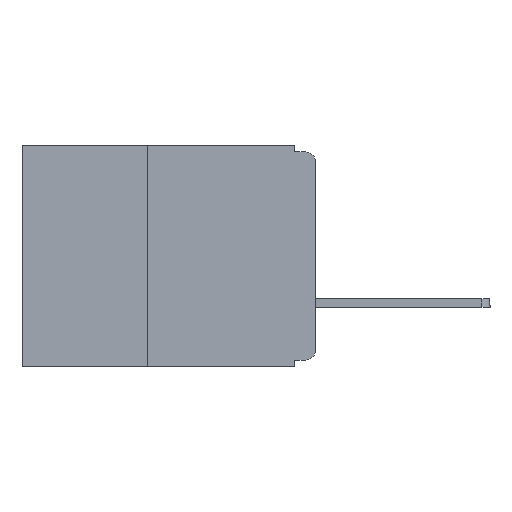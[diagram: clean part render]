
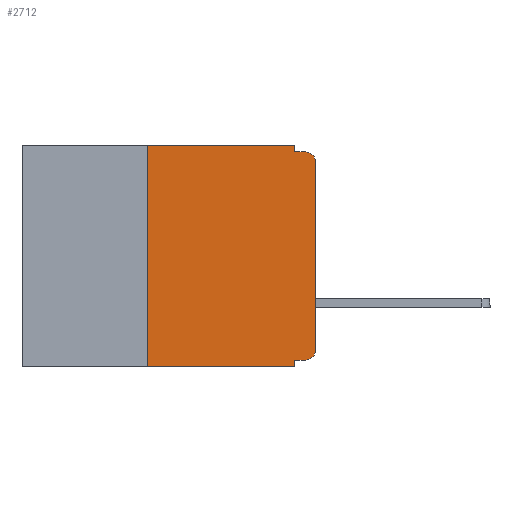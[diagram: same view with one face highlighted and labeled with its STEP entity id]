
A CAD part, left-side view. The second image highlights one B-rep face of the part: STEP entity #2712.
In plain terms, the highlighted planar face has unit normal (-1, 0, 0).
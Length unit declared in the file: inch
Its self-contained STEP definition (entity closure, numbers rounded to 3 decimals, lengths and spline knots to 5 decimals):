
#52 = VECTOR ( 'NONE', #12586, 39.37008 ) ;
#129 = ORIENTED_EDGE ( 'NONE', *, *, #21061, .T. ) ;
#173 = CARTESIAN_POINT ( 'NONE',  ( 0., 0.437, -0.33 ) ) ;
#361 = CARTESIAN_POINT ( 'NONE',  ( 0., 0., -0.305 ) ) ;
#494 = EDGE_CURVE ( 'NONE', #7946, #4971, #5809, .T. ) ;
#537 = EDGE_CURVE ( 'NONE', #8335, #21397, #9353, .T. ) ;
#697 = LINE ( 'NONE', #15711, #18582 ) ;
#946 = EDGE_LOOP ( 'NONE', ( #16681, #20934, #6459, #18796, #12534, #5218, #9068, #18330, #2306, #129 ) ) ;
#1603 = LINE ( 'NONE', #14274, #14905 ) ;
#1838 = DIRECTION ( 'NONE',  ( 0., 0., -1. ) ) ;
#2045 = VERTEX_POINT ( 'NONE', #22030 ) ;
#2090 = CARTESIAN_POINT ( 'NONE',  ( 0., 0.25, 0. ) ) ;
#2243 = CARTESIAN_POINT ( 'NONE',  ( 0., 0.031, -0.32 ) ) ;
#2306 = ORIENTED_EDGE ( 'NONE', *, *, #6783, .F. ) ;
#2453 = EDGE_CURVE ( 'NONE', #14867, #21746, #14072, .T. ) ;
#2712 = ADVANCED_FACE ( 'NONE', ( #4031 ), #21261, .F. ) ;
#3040 = VERTEX_POINT ( 'NONE', #17098 ) ;
#3292 = VECTOR ( 'NONE', #3670, 39.37008 ) ;
#3362 = AXIS2_PLACEMENT_3D ( 'NONE', #14103, #13727, #13540 ) ;
#3487 = LINE ( 'NONE', #14834, #12226 ) ;
#3670 = DIRECTION ( 'NONE',  ( 0., -1., 0. ) ) ;
#4031 = FACE_OUTER_BOUND ( 'NONE', #946, .T. ) ;
#4135 = CARTESIAN_POINT ( 'NONE',  ( 0., 0.015, -0.01 ) ) ;
#4971 = VERTEX_POINT ( 'NONE', #4135 ) ;
#5218 = ORIENTED_EDGE ( 'NONE', *, *, #537, .F. ) ;
#5604 = CARTESIAN_POINT ( 'NONE',  ( 0., 0., -0.32 ) ) ;
#5809 = CIRCLE ( 'NONE', #3362, 0.015 ) ;
#6049 = VECTOR ( 'NONE', #6880, 39.37008 ) ;
#6459 = ORIENTED_EDGE ( 'NONE', *, *, #9477, .F. ) ;
#6531 = CARTESIAN_POINT ( 'NONE',  ( 0., 0.031, -0.01 ) ) ;
#6783 = EDGE_CURVE ( 'NONE', #2045, #14867, #19770, .T. ) ;
#6880 = DIRECTION ( 'NONE',  ( 0., 0., 1. ) ) ;
#7089 = CARTESIAN_POINT ( 'NONE',  ( 0., 0.031, -0.33 ) ) ;
#7946 = VERTEX_POINT ( 'NONE', #16350 ) ;
#7999 = LINE ( 'NONE', #173, #3292 ) ;
#8028 = EDGE_CURVE ( 'NONE', #3040, #13187, #3487, .T. ) ;
#8335 = VERTEX_POINT ( 'NONE', #10473 ) ;
#9068 = ORIENTED_EDGE ( 'NONE', *, *, #12795, .T. ) ;
#9353 = LINE ( 'NONE', #11539, #52 ) ;
#9477 = EDGE_CURVE ( 'NONE', #13187, #4971, #697, .T. ) ;
#9934 = CARTESIAN_POINT ( 'NONE',  ( 0., 0.015, -0.305 ) ) ;
#10473 = CARTESIAN_POINT ( 'NONE',  ( 0., 0.25, -0.33 ) ) ;
#10648 = LINE ( 'NONE', #12018, #6049 ) ;
#11206 = CARTESIAN_POINT ( 'NONE',  ( 0., 0.031, -0.33 ) ) ;
#11539 = CARTESIAN_POINT ( 'NONE',  ( 0., 0.25, -0.33 ) ) ;
#11648 = DIRECTION ( 'NONE',  ( 0., 0., -1. ) ) ;
#11749 = VERTEX_POINT ( 'NONE', #361 ) ;
#12018 = CARTESIAN_POINT ( 'NONE',  ( 0., 0., 0. ) ) ;
#12226 = VECTOR ( 'NONE', #16586, 39.37008 ) ;
#12534 = ORIENTED_EDGE ( 'NONE', *, *, #14180, .F. ) ;
#12586 = DIRECTION ( 'NONE',  ( 0., 0., 1. ) ) ;
#12795 = EDGE_CURVE ( 'NONE', #8335, #21746, #7999, .T. ) ;
#13187 = VERTEX_POINT ( 'NONE', #6531 ) ;
#13533 = VECTOR ( 'NONE', #1838, 39.37008 ) ;
#13540 = DIRECTION ( 'NONE',  ( 0., 0., -1. ) ) ;
#13727 = DIRECTION ( 'NONE',  ( -1., 0., 0. ) ) ;
#14072 = LINE ( 'NONE', #7089, #13533 ) ;
#14103 = CARTESIAN_POINT ( 'NONE',  ( 0., 0.015, -0.025 ) ) ;
#14180 = EDGE_CURVE ( 'NONE', #21397, #3040, #1603, .T. ) ;
#14274 = CARTESIAN_POINT ( 'NONE',  ( 0., 0.437, 0. ) ) ;
#14684 = VECTOR ( 'NONE', #19457, 39.37008 ) ;
#14834 = CARTESIAN_POINT ( 'NONE',  ( 0., 0.031, 0. ) ) ;
#14867 = VERTEX_POINT ( 'NONE', #2243 ) ;
#14905 = VECTOR ( 'NONE', #16042, 39.37008 ) ;
#14994 = CIRCLE ( 'NONE', #15205, 0.015 ) ;
#15205 = AXIS2_PLACEMENT_3D ( 'NONE', #9934, #21839, #11648 ) ;
#15711 = CARTESIAN_POINT ( 'NONE',  ( 0., 0., -0.01 ) ) ;
#16042 = DIRECTION ( 'NONE',  ( 0., -1., 0. ) ) ;
#16350 = CARTESIAN_POINT ( 'NONE',  ( 0., 0., -0.025 ) ) ;
#16586 = DIRECTION ( 'NONE',  ( 0., 0., -1. ) ) ;
#16681 = ORIENTED_EDGE ( 'NONE', *, *, #22037, .T. ) ;
#17098 = CARTESIAN_POINT ( 'NONE',  ( 0., 0.031, 0. ) ) ;
#18330 = ORIENTED_EDGE ( 'NONE', *, *, #2453, .F. ) ;
#18582 = VECTOR ( 'NONE', #19106, 39.37008 ) ;
#18796 = ORIENTED_EDGE ( 'NONE', *, *, #8028, .F. ) ;
#19106 = DIRECTION ( 'NONE',  ( 0., -1., 0. ) ) ;
#19457 = DIRECTION ( 'NONE',  ( 0., 1., 0. ) ) ;
#19770 = LINE ( 'NONE', #5604, #14684 ) ;
#20934 = ORIENTED_EDGE ( 'NONE', *, *, #494, .T. ) ;
#21061 = EDGE_CURVE ( 'NONE', #2045, #11749, #14994, .T. ) ;
#21108 = DIRECTION ( 'NONE',  ( 1., 0., 0. ) ) ;
#21186 = CARTESIAN_POINT ( 'NONE',  ( 0., 0.437, 0. ) ) ;
#21261 = PLANE ( 'NONE',  #22276 ) ;
#21397 = VERTEX_POINT ( 'NONE', #2090 ) ;
#21746 = VERTEX_POINT ( 'NONE', #11206 ) ;
#21839 = DIRECTION ( 'NONE',  ( -1., 0., 0. ) ) ;
#21990 = DIRECTION ( 'NONE',  ( 0., 0., -1. ) ) ;
#22030 = CARTESIAN_POINT ( 'NONE',  ( 0., 0.015, -0.32 ) ) ;
#22037 = EDGE_CURVE ( 'NONE', #11749, #7946, #10648, .T. ) ;
#22276 = AXIS2_PLACEMENT_3D ( 'NONE', #21186, #21108, #21990 ) ;
